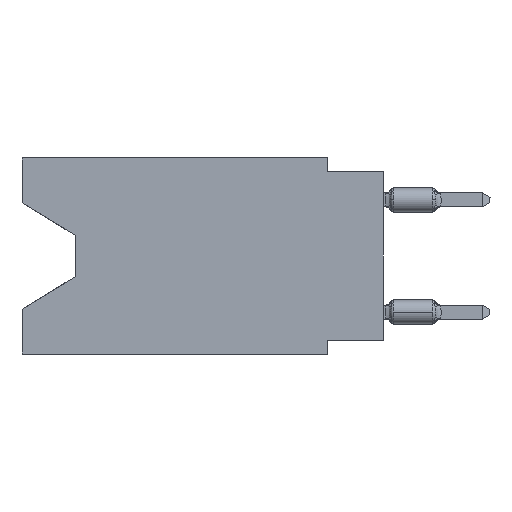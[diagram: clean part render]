
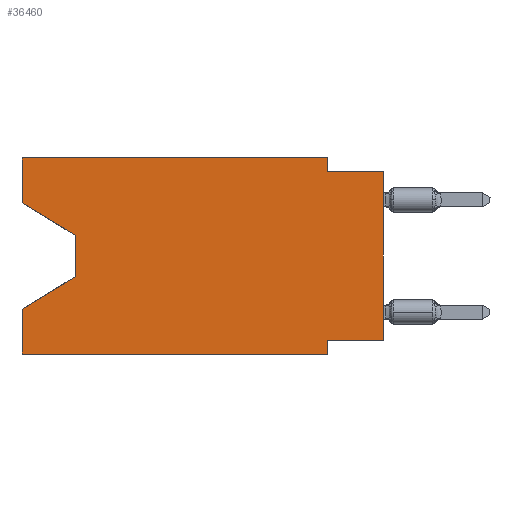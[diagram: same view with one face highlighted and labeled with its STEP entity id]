
A CAD part, left-side view. The second image highlights one B-rep face of the part: STEP entity #36460.
In plain terms, the highlighted planar face has unit normal (-1, 0, 0).
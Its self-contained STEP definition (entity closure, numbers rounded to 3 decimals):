
#19 = CARTESIAN_POINT ( 'NONE',  ( 0., 16.383, -8.89 ) ) ;
#1189 = DIRECTION ( 'NONE',  ( 0., 0., 1. ) ) ;
#1276 = LINE ( 'NONE', #30329, #38501 ) ;
#1874 = CARTESIAN_POINT ( 'NONE',  ( 0., 2.54, -0.635 ) ) ;
#2383 = ORIENTED_EDGE ( 'NONE', *, *, #12844, .T. ) ;
#2748 = VERTEX_POINT ( 'NONE', #44406 ) ;
#3130 = CARTESIAN_POINT ( 'NONE',  ( 0., 2.54, -8.89 ) ) ;
#3201 = CARTESIAN_POINT ( 'NONE',  ( 0., 16.383, 0. ) ) ;
#3479 = VERTEX_POINT ( 'NONE', #13593 ) ;
#3755 = VERTEX_POINT ( 'NONE', #18929 ) ;
#3894 = VECTOR ( 'NONE', #1189, 1000. ) ;
#5022 = ORIENTED_EDGE ( 'NONE', *, *, #23339, .T. ) ;
#5776 = CARTESIAN_POINT ( 'NONE',  ( 0., 0., 0. ) ) ;
#6106 = EDGE_CURVE ( 'NONE', #7819, #37332, #52791, .T. ) ;
#6474 = DIRECTION ( 'NONE',  ( 0., 0., -1. ) ) ;
#6875 = VECTOR ( 'NONE', #14469, 1000. ) ;
#7225 = EDGE_CURVE ( 'NONE', #18677, #41305, #43078, .T. ) ;
#7819 = VERTEX_POINT ( 'NONE', #38975 ) ;
#7952 = DIRECTION ( 'NONE',  ( 0., 0.855, -0.519 ) ) ;
#8730 = CARTESIAN_POINT ( 'NONE',  ( 0., 16.383, 0. ) ) ;
#8982 = VECTOR ( 'NONE', #29290, 1000. ) ;
#11359 = FACE_OUTER_BOUND ( 'NONE', #44680, .T. ) ;
#12269 = ORIENTED_EDGE ( 'NONE', *, *, #7225, .F. ) ;
#12844 = EDGE_CURVE ( 'NONE', #2748, #23067, #21551, .T. ) ;
#13403 = VERTEX_POINT ( 'NONE', #41742 ) ;
#13593 = CARTESIAN_POINT ( 'NONE',  ( 0., 13.97, -3.505 ) ) ;
#14469 = DIRECTION ( 'NONE',  ( 0., -1., 0. ) ) ;
#16046 = DIRECTION ( 'NONE',  ( 0., -1., 0. ) ) ;
#17555 = CARTESIAN_POINT ( 'NONE',  ( 0., 2.54, 0. ) ) ;
#17739 = EDGE_CURVE ( 'NONE', #23557, #3755, #25031, .T. ) ;
#18064 = VECTOR ( 'NONE', #30045, 1000. ) ;
#18174 = VECTOR ( 'NONE', #25304, 1000. ) ;
#18351 = LINE ( 'NONE', #34112, #40105 ) ;
#18677 = VERTEX_POINT ( 'NONE', #43343 ) ;
#18700 = LINE ( 'NONE', #3201, #48001 ) ;
#18929 = CARTESIAN_POINT ( 'NONE',  ( 0., 16.383, 0. ) ) ;
#19191 = EDGE_CURVE ( 'NONE', #41305, #23067, #23446, .T. ) ;
#19992 = ORIENTED_EDGE ( 'NONE', *, *, #32301, .F. ) ;
#21551 = LINE ( 'NONE', #5776, #3894 ) ;
#22999 = CARTESIAN_POINT ( 'NONE',  ( 0., 0., -8.255 ) ) ;
#23067 = VERTEX_POINT ( 'NONE', #36109 ) ;
#23339 = EDGE_CURVE ( 'NONE', #3479, #7819, #46396, .T. ) ;
#23446 = LINE ( 'NONE', #31312, #6875 ) ;
#23557 = VERTEX_POINT ( 'NONE', #41698 ) ;
#23796 = EDGE_CURVE ( 'NONE', #42028, #40696, #37231, .T. ) ;
#24471 = ORIENTED_EDGE ( 'NONE', *, *, #48442, .F. ) ;
#24623 = VECTOR ( 'NONE', #50256, 1000. ) ;
#24938 = AXIS2_PLACEMENT_3D ( 'NONE', #44488, #51857, #6474 ) ;
#25029 = ORIENTED_EDGE ( 'NONE', *, *, #23796, .T. ) ;
#25031 = LINE ( 'NONE', #8730, #18174 ) ;
#25304 = DIRECTION ( 'NONE',  ( 0., 0., 1. ) ) ;
#27623 = ORIENTED_EDGE ( 'NONE', *, *, #47057, .T. ) ;
#27662 = PLANE ( 'NONE',  #24938 ) ;
#27872 = EDGE_CURVE ( 'NONE', #42028, #37332, #18700, .T. ) ;
#28189 = DIRECTION ( 'NONE',  ( 0., 0., 1. ) ) ;
#29290 = DIRECTION ( 'NONE',  ( 0., 0., -1. ) ) ;
#30045 = DIRECTION ( 'NONE',  ( 0., 0., -1. ) ) ;
#30329 = CARTESIAN_POINT ( 'NONE',  ( 0., 2.54, -8.89 ) ) ;
#31312 = CARTESIAN_POINT ( 'NONE',  ( 0., 0., -0.635 ) ) ;
#31588 = CARTESIAN_POINT ( 'NONE',  ( 0., 13.97, -5.385 ) ) ;
#32061 = ORIENTED_EDGE ( 'NONE', *, *, #19191, .F. ) ;
#32301 = EDGE_CURVE ( 'NONE', #2748, #13403, #35495, .T. ) ;
#33463 = VECTOR ( 'NONE', #16046, 1000. ) ;
#34112 = CARTESIAN_POINT ( 'NONE',  ( 0., 16.383, -2.038 ) ) ;
#35495 = LINE ( 'NONE', #22999, #49067 ) ;
#36109 = CARTESIAN_POINT ( 'NONE',  ( 0., 0., -0.635 ) ) ;
#36460 = ADVANCED_FACE ( 'NONE', ( #11359 ), #27662, .F. ) ;
#36701 = LINE ( 'NONE', #45385, #33463 ) ;
#36852 = ORIENTED_EDGE ( 'NONE', *, *, #27872, .F. ) ;
#37231 = LINE ( 'NONE', #19, #24623 ) ;
#37332 = VERTEX_POINT ( 'NONE', #47356 ) ;
#38501 = VECTOR ( 'NONE', #46624, 1000. ) ;
#38975 = CARTESIAN_POINT ( 'NONE',  ( 0., 13.97, -5.385 ) ) ;
#40105 = VECTOR ( 'NONE', #47715, 1000. ) ;
#40653 = ORIENTED_EDGE ( 'NONE', *, *, #6106, .T. ) ;
#40696 = VERTEX_POINT ( 'NONE', #3130 ) ;
#41305 = VERTEX_POINT ( 'NONE', #1874 ) ;
#41698 = CARTESIAN_POINT ( 'NONE',  ( 0., 16.383, -2.038 ) ) ;
#41742 = CARTESIAN_POINT ( 'NONE',  ( 0., 2.54, -8.255 ) ) ;
#42028 = VERTEX_POINT ( 'NONE', #50645 ) ;
#43078 = LINE ( 'NONE', #17555, #18064 ) ;
#43343 = CARTESIAN_POINT ( 'NONE',  ( 0., 2.54, 0. ) ) ;
#43917 = VECTOR ( 'NONE', #7952, 1000. ) ;
#44238 = ORIENTED_EDGE ( 'NONE', *, *, #50642, .F. ) ;
#44406 = CARTESIAN_POINT ( 'NONE',  ( 0., 0., -8.255 ) ) ;
#44488 = CARTESIAN_POINT ( 'NONE',  ( 0., 16.383, 0. ) ) ;
#44680 = EDGE_LOOP ( 'NONE', ( #27623, #5022, #40653, #36852, #25029, #24471, #19992, #2383, #32061, #12269, #44238, #53161 ) ) ;
#45385 = CARTESIAN_POINT ( 'NONE',  ( 0., 16.383, 0. ) ) ;
#46396 = LINE ( 'NONE', #49945, #8982 ) ;
#46624 = DIRECTION ( 'NONE',  ( 0., 0., -1. ) ) ;
#47057 = EDGE_CURVE ( 'NONE', #23557, #3479, #18351, .T. ) ;
#47356 = CARTESIAN_POINT ( 'NONE',  ( 0., 16.383, -6.852 ) ) ;
#47715 = DIRECTION ( 'NONE',  ( 0., -0.855, -0.519 ) ) ;
#48001 = VECTOR ( 'NONE', #28189, 1000. ) ;
#48442 = EDGE_CURVE ( 'NONE', #13403, #40696, #1276, .T. ) ;
#49067 = VECTOR ( 'NONE', #51539, 1000. ) ;
#49945 = CARTESIAN_POINT ( 'NONE',  ( 0., 13.97, -3.505 ) ) ;
#50256 = DIRECTION ( 'NONE',  ( 0., -1., 0. ) ) ;
#50642 = EDGE_CURVE ( 'NONE', #3755, #18677, #36701, .T. ) ;
#50645 = CARTESIAN_POINT ( 'NONE',  ( 0., 16.383, -8.89 ) ) ;
#51539 = DIRECTION ( 'NONE',  ( 0., 1., 0. ) ) ;
#51857 = DIRECTION ( 'NONE',  ( 1., 0., 0. ) ) ;
#52791 = LINE ( 'NONE', #31588, #43917 ) ;
#53161 = ORIENTED_EDGE ( 'NONE', *, *, #17739, .F. ) ;
